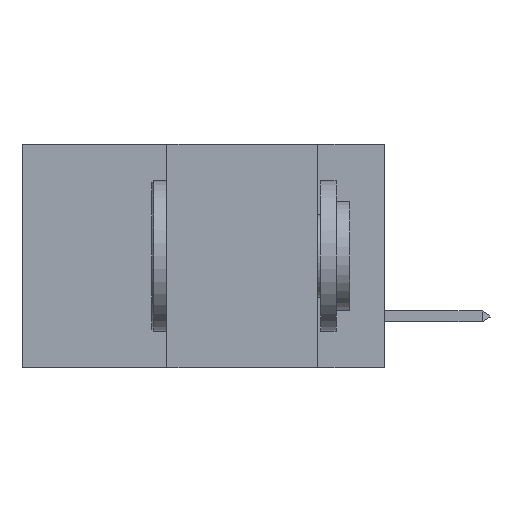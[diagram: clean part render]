
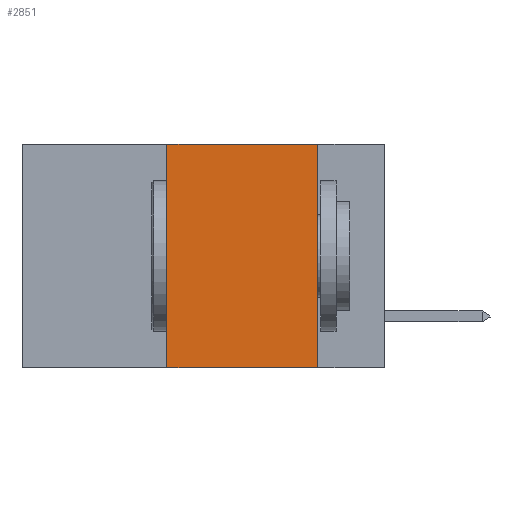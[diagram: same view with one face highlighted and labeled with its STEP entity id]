
A CAD part, left-side view. The second image highlights one B-rep face of the part: STEP entity #2851.
In plain terms, the highlighted planar face has unit normal (-1, 0, 0).
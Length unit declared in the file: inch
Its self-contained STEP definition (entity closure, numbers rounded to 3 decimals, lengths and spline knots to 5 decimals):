
#402 = VECTOR ( 'NONE', #18986, 39.37008 ) ;
#480 = VERTEX_POINT ( 'NONE', #8741 ) ;
#1939 = CARTESIAN_POINT ( 'NONE',  ( 0., 0.36, -0.37 ) ) ;
#2224 = CARTESIAN_POINT ( 'NONE',  ( 0., 0.6, -0.37 ) ) ;
#2851 = ADVANCED_FACE ( 'NONE', ( #5084 ), #22920, .F. ) ;
#3001 = EDGE_LOOP ( 'NONE', ( #8136, #9302, #19630, #20171 ) ) ;
#3276 = CARTESIAN_POINT ( 'NONE',  ( 0., 0.36, 0. ) ) ;
#3430 = EDGE_CURVE ( 'NONE', #480, #13606, #7694, .T. ) ;
#3872 = DIRECTION ( 'NONE',  ( 0., 0., -1. ) ) ;
#3904 = DIRECTION ( 'NONE',  ( 1., 0., 0. ) ) ;
#4264 = LINE ( 'NONE', #17944, #14852 ) ;
#4301 = CARTESIAN_POINT ( 'NONE',  ( 0., 0.6, 0. ) ) ;
#5084 = FACE_OUTER_BOUND ( 'NONE', #3001, .T. ) ;
#5669 = DIRECTION ( 'NONE',  ( 0., 0., -1. ) ) ;
#6835 = DIRECTION ( 'NONE',  ( 0., 0., 1. ) ) ;
#6866 = LINE ( 'NONE', #11832, #20869 ) ;
#7694 = LINE ( 'NONE', #23266, #12675 ) ;
#8136 = ORIENTED_EDGE ( 'NONE', *, *, #3430, .F. ) ;
#8180 = AXIS2_PLACEMENT_3D ( 'NONE', #4301, #3904, #3872 ) ;
#8741 = CARTESIAN_POINT ( 'NONE',  ( 0., 0.11, 0. ) ) ;
#9302 = ORIENTED_EDGE ( 'NONE', *, *, #17556, .F. ) ;
#11832 = CARTESIAN_POINT ( 'NONE',  ( 0., 0.6, 0. ) ) ;
#12675 = VECTOR ( 'NONE', #5669, 39.37008 ) ;
#13606 = VERTEX_POINT ( 'NONE', #22769 ) ;
#13675 = DIRECTION ( 'NONE',  ( 0., -1., 0. ) ) ;
#14852 = VECTOR ( 'NONE', #6835, 39.37008 ) ;
#15570 = EDGE_CURVE ( 'NONE', #19634, #20025, #4264, .T. ) ;
#17556 = EDGE_CURVE ( 'NONE', #20025, #480, #6866, .T. ) ;
#17944 = CARTESIAN_POINT ( 'NONE',  ( 0., 0.36, 0. ) ) ;
#18986 = DIRECTION ( 'NONE',  ( 0., -1., 0. ) ) ;
#19630 = ORIENTED_EDGE ( 'NONE', *, *, #15570, .F. ) ;
#19634 = VERTEX_POINT ( 'NONE', #1939 ) ;
#20025 = VERTEX_POINT ( 'NONE', #3276 ) ;
#20171 = ORIENTED_EDGE ( 'NONE', *, *, #20919, .T. ) ;
#20193 = LINE ( 'NONE', #2224, #402 ) ;
#20869 = VECTOR ( 'NONE', #13675, 39.37008 ) ;
#20919 = EDGE_CURVE ( 'NONE', #19634, #13606, #20193, .T. ) ;
#22769 = CARTESIAN_POINT ( 'NONE',  ( 0., 0.11, -0.37 ) ) ;
#22920 = PLANE ( 'NONE',  #8180 ) ;
#23266 = CARTESIAN_POINT ( 'NONE',  ( 0., 0.11, 0. ) ) ;
